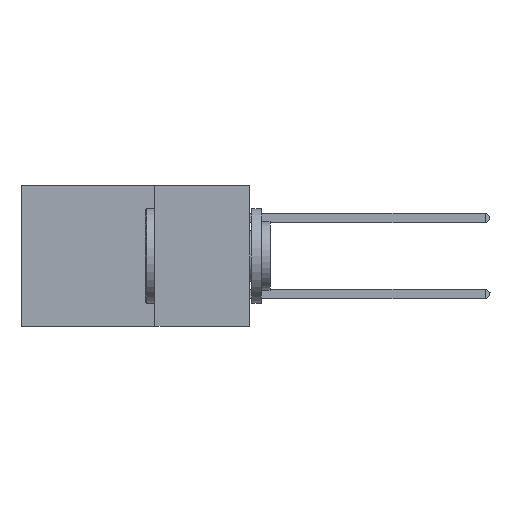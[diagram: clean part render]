
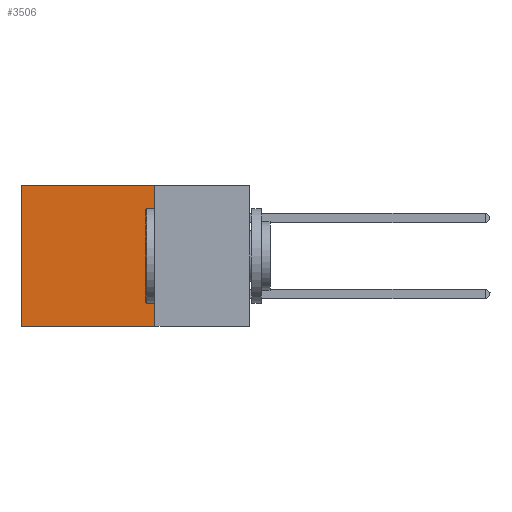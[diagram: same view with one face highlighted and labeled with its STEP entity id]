
A CAD part, left-side view. The second image highlights one B-rep face of the part: STEP entity #3506.
In plain terms, the highlighted planar face has unit normal (-1, 0, 0).
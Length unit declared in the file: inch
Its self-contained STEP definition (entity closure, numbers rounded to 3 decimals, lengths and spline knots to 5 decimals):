
#2028 = DIRECTION ( 'NONE',  ( 0., 0., -1. ) ) ;
#2059 = VECTOR ( 'NONE', #12885, 39.37008 ) ;
#2329 = ORIENTED_EDGE ( 'NONE', *, *, #16593, .F. ) ;
#3506 = ADVANCED_FACE ( 'NONE', ( #5000 ), #23934, .F. ) ;
#3543 = LINE ( 'NONE', #10216, #24123 ) ;
#4460 = CARTESIAN_POINT ( 'NONE',  ( 0.2875, 0.25, -0.37 ) ) ;
#5000 = FACE_OUTER_BOUND ( 'NONE', #11099, .T. ) ;
#6549 = ORIENTED_EDGE ( 'NONE', *, *, #23124, .F. ) ;
#6893 = CARTESIAN_POINT ( 'NONE',  ( 0.2875, 0.6, -0.37 ) ) ;
#7858 = VERTEX_POINT ( 'NONE', #6893 ) ;
#8818 = EDGE_CURVE ( 'NONE', #23731, #21368, #9955, .T. ) ;
#9929 = DIRECTION ( 'NONE',  ( 0., 0., -1. ) ) ;
#9955 = LINE ( 'NONE', #15827, #10892 ) ;
#10216 = CARTESIAN_POINT ( 'NONE',  ( 0.2875, 0.25, 0. ) ) ;
#10892 = VECTOR ( 'NONE', #13999, 39.37008 ) ;
#11084 = AXIS2_PLACEMENT_3D ( 'NONE', #11960, #15838, #25733 ) ;
#11099 = EDGE_LOOP ( 'NONE', ( #13825, #2329, #6549, #14985 ) ) ;
#11751 = CARTESIAN_POINT ( 'NONE',  ( 0.2875, 0.6, 0. ) ) ;
#11960 = CARTESIAN_POINT ( 'NONE',  ( 0.2875, 0.25, 0. ) ) ;
#12197 = CARTESIAN_POINT ( 'NONE',  ( 0.2875, 0.25, 0. ) ) ;
#12885 = DIRECTION ( 'NONE',  ( 0., 1., 0. ) ) ;
#13045 = VECTOR ( 'NONE', #9929, 39.37008 ) ;
#13825 = ORIENTED_EDGE ( 'NONE', *, *, #14959, .T. ) ;
#13999 = DIRECTION ( 'NONE',  ( 0., 1., 0. ) ) ;
#14959 = EDGE_CURVE ( 'NONE', #21368, #7858, #20251, .T. ) ;
#14985 = ORIENTED_EDGE ( 'NONE', *, *, #8818, .T. ) ;
#15169 = CARTESIAN_POINT ( 'NONE',  ( 0.2875, 0.25, -0.37 ) ) ;
#15827 = CARTESIAN_POINT ( 'NONE',  ( 0.2875, 0.25, 0. ) ) ;
#15838 = DIRECTION ( 'NONE',  ( 1., 0., 0. ) ) ;
#16593 = EDGE_CURVE ( 'NONE', #20300, #7858, #22949, .T. ) ;
#20251 = LINE ( 'NONE', #11751, #13045 ) ;
#20300 = VERTEX_POINT ( 'NONE', #4460 ) ;
#21368 = VERTEX_POINT ( 'NONE', #24121 ) ;
#22949 = LINE ( 'NONE', #15169, #2059 ) ;
#23124 = EDGE_CURVE ( 'NONE', #23731, #20300, #3543, .T. ) ;
#23731 = VERTEX_POINT ( 'NONE', #12197 ) ;
#23934 = PLANE ( 'NONE',  #11084 ) ;
#24121 = CARTESIAN_POINT ( 'NONE',  ( 0.2875, 0.6, 0. ) ) ;
#24123 = VECTOR ( 'NONE', #2028, 39.37008 ) ;
#25733 = DIRECTION ( 'NONE',  ( 0., 0., -1. ) ) ;
